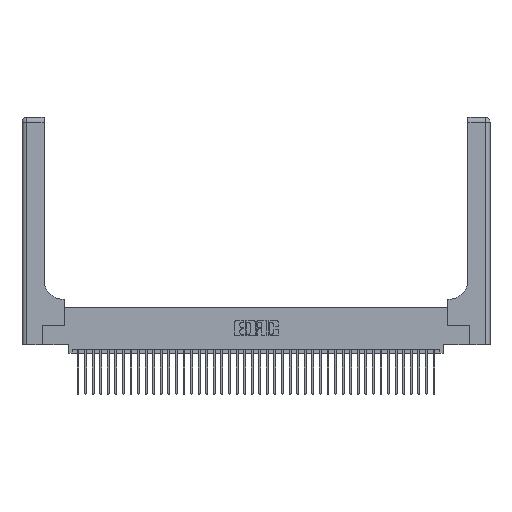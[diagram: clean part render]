
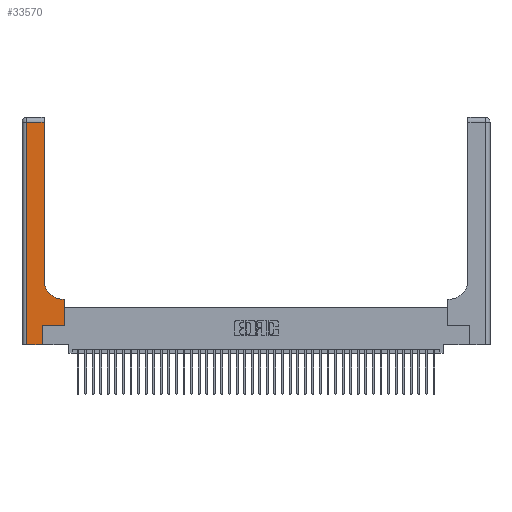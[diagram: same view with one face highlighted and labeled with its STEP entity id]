
A CAD part, top view. The second image highlights one B-rep face of the part: STEP entity #33570.
In plain terms, the highlighted planar face has unit normal (0, 0, 1).
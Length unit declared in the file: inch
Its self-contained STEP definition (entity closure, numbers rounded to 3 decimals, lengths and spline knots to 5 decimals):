
#93 = VERTEX_POINT ( 'NONE', #7485 ) ;
#631 = DIRECTION ( 'NONE',  ( 1., 0., 0. ) ) ;
#1165 = VERTEX_POINT ( 'NONE', #25961 ) ;
#1256 = DIRECTION ( 'NONE',  ( -1., 0., 0. ) ) ;
#1516 = EDGE_CURVE ( 'NONE', #13590, #6796, #28734, .T. ) ;
#1577 = LINE ( 'NONE', #2477, #35289 ) ;
#1855 = CARTESIAN_POINT ( 'NONE',  ( 0., 3., 0.37 ) ) ;
#2379 = VERTEX_POINT ( 'NONE', #28884 ) ;
#2382 = EDGE_CURVE ( 'NONE', #1165, #21944, #1577, .T. ) ;
#2477 = CARTESIAN_POINT ( 'NONE',  ( 0.5585, 0.25, 0.37 ) ) ;
#4199 = EDGE_CURVE ( 'NONE', #93, #40086, #30532, .T. ) ;
#4384 = DIRECTION ( 'NONE',  ( 1., 0., 0. ) ) ;
#4385 = CARTESIAN_POINT ( 'NONE',  ( 0.5415, 0.85, 0.37 ) ) ;
#5117 = PLANE ( 'NONE',  #16930 ) ;
#6017 = CARTESIAN_POINT ( 'NONE',  ( 0.269, 0., 0.37 ) ) ;
#6796 = VERTEX_POINT ( 'NONE', #36665 ) ;
#7485 = CARTESIAN_POINT ( 'NONE',  ( 0.06, 0., 0.37 ) ) ;
#7647 = DIRECTION ( 'NONE',  ( 1., 0., 0. ) ) ;
#8275 = ORIENTED_EDGE ( 'NONE', *, *, #4199, .T. ) ;
#8406 = LINE ( 'NONE', #6017, #34479 ) ;
#8407 = DIRECTION ( 'NONE',  ( 0., 0., -1. ) ) ;
#8530 = EDGE_CURVE ( 'NONE', #40086, #14388, #8406, .T. ) ;
#8952 = CARTESIAN_POINT ( 'NONE',  ( 0., 2.94, 0.37 ) ) ;
#10056 = CARTESIAN_POINT ( 'NONE',  ( 0.269, 0.25, 0.37 ) ) ;
#10411 = ORIENTED_EDGE ( 'NONE', *, *, #25465, .T. ) ;
#10464 = CARTESIAN_POINT ( 'NONE',  ( 0., 0., 0.37 ) ) ;
#11373 = CARTESIAN_POINT ( 'NONE',  ( 0.2915, 3., 0.37 ) ) ;
#11692 = CARTESIAN_POINT ( 'NONE',  ( 0.5415, 0.6, 0.37 ) ) ;
#12068 = EDGE_CURVE ( 'NONE', #21486, #13590, #19821, .T. ) ;
#13590 = VERTEX_POINT ( 'NONE', #35259 ) ;
#13785 = LINE ( 'NONE', #15949, #38807 ) ;
#14089 = CARTESIAN_POINT ( 'NONE',  ( 0.5585, 0.6, 0.37 ) ) ;
#14388 = VERTEX_POINT ( 'NONE', #10056 ) ;
#15949 = CARTESIAN_POINT ( 'NONE',  ( 0.06, 3., 0.37 ) ) ;
#16930 = AXIS2_PLACEMENT_3D ( 'NONE', #1855, #8407, #31253 ) ;
#17801 = DIRECTION ( 'NONE',  ( 0., 1., 0. ) ) ;
#17869 = ORIENTED_EDGE ( 'NONE', *, *, #27491, .T. ) ;
#18253 = LINE ( 'NONE', #20643, #19276 ) ;
#19229 = DIRECTION ( 'NONE',  ( 0., -1., 0. ) ) ;
#19276 = VECTOR ( 'NONE', #4384, 39.37008 ) ;
#19395 = VECTOR ( 'NONE', #1256, 39.37008 ) ;
#19726 = ORIENTED_EDGE ( 'NONE', *, *, #2382, .T. ) ;
#19821 = CIRCLE ( 'NONE', #40285, 0.25 ) ;
#20643 = CARTESIAN_POINT ( 'NONE',  ( 0.269, 0.25, 0.37 ) ) ;
#21486 = VERTEX_POINT ( 'NONE', #11692 ) ;
#21944 = VERTEX_POINT ( 'NONE', #14089 ) ;
#22223 = ORIENTED_EDGE ( 'NONE', *, *, #1516, .T. ) ;
#22447 = ORIENTED_EDGE ( 'NONE', *, *, #12068, .T. ) ;
#25465 = EDGE_CURVE ( 'NONE', #14388, #1165, #18253, .T. ) ;
#25961 = CARTESIAN_POINT ( 'NONE',  ( 0.5585, 0.25, 0.37 ) ) ;
#26847 = FACE_OUTER_BOUND ( 'NONE', #31227, .T. ) ;
#27202 = DIRECTION ( 'NONE',  ( 0., 0., -1. ) ) ;
#27491 = EDGE_CURVE ( 'NONE', #6796, #2379, #36894, .T. ) ;
#27682 = VECTOR ( 'NONE', #17801, 39.37008 ) ;
#28061 = LINE ( 'NONE', #33787, #19395 ) ;
#28734 = LINE ( 'NONE', #11373, #27682 ) ;
#28884 = CARTESIAN_POINT ( 'NONE',  ( 0.06, 2.94, 0.37 ) ) ;
#29748 = EDGE_CURVE ( 'NONE', #21944, #21486, #28061, .T. ) ;
#30532 = LINE ( 'NONE', #10464, #37153 ) ;
#31227 = EDGE_LOOP ( 'NONE', ( #22223, #17869, #34530, #8275, #34370, #10411, #19726, #41301, #22447 ) ) ;
#31253 = DIRECTION ( 'NONE',  ( -1., 0., 0. ) ) ;
#32161 = DIRECTION ( 'NONE',  ( 0., 1., 0. ) ) ;
#33570 = ADVANCED_FACE ( 'NONE', ( #26847 ), #5117, .F. ) ;
#33787 = CARTESIAN_POINT ( 'NONE',  ( 0.2915, 0.6, 0.37 ) ) ;
#34370 = ORIENTED_EDGE ( 'NONE', *, *, #8530, .T. ) ;
#34479 = VECTOR ( 'NONE', #32161, 39.37008 ) ;
#34530 = ORIENTED_EDGE ( 'NONE', *, *, #37682, .T. ) ;
#35259 = CARTESIAN_POINT ( 'NONE',  ( 0.2915, 0.85, 0.37 ) ) ;
#35289 = VECTOR ( 'NONE', #35446, 39.37008 ) ;
#35446 = DIRECTION ( 'NONE',  ( 0., 1., 0. ) ) ;
#35888 = VECTOR ( 'NONE', #41430, 39.37008 ) ;
#36665 = CARTESIAN_POINT ( 'NONE',  ( 0.2915, 2.94, 0.37 ) ) ;
#36894 = LINE ( 'NONE', #8952, #35888 ) ;
#37153 = VECTOR ( 'NONE', #631, 39.37008 ) ;
#37682 = EDGE_CURVE ( 'NONE', #2379, #93, #13785, .T. ) ;
#38807 = VECTOR ( 'NONE', #19229, 39.37008 ) ;
#38977 = CARTESIAN_POINT ( 'NONE',  ( 0.269, 0., 0.37 ) ) ;
#40086 = VERTEX_POINT ( 'NONE', #38977 ) ;
#40285 = AXIS2_PLACEMENT_3D ( 'NONE', #4385, #27202, #7647 ) ;
#41301 = ORIENTED_EDGE ( 'NONE', *, *, #29748, .T. ) ;
#41430 = DIRECTION ( 'NONE',  ( -1., 0., 0. ) ) ;
